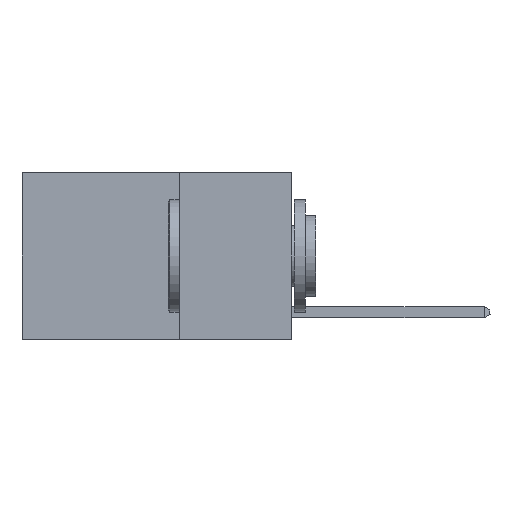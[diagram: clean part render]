
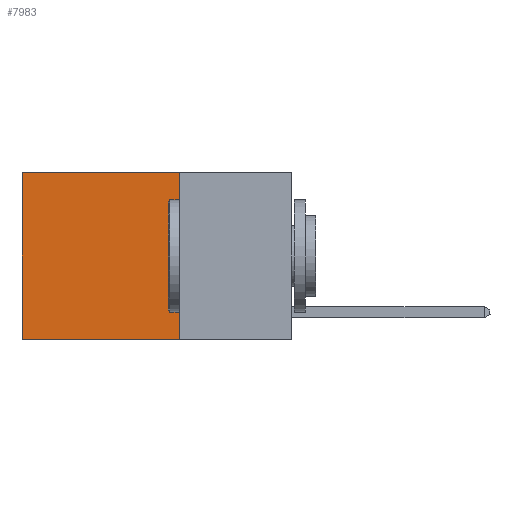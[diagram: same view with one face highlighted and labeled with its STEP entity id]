
A CAD part, left-side view. The second image highlights one B-rep face of the part: STEP entity #7983.
In plain terms, the highlighted planar face has unit normal (-1, 0, 0).
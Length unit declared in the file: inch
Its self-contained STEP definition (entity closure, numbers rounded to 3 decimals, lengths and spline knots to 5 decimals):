
#146 = VECTOR ( 'NONE', #8504, 39.37008 ) ;
#1455 = LINE ( 'NONE', #8732, #4046 ) ;
#1481 = DIRECTION ( 'NONE',  ( 0., 0., -1. ) ) ;
#2478 = CARTESIAN_POINT ( 'NONE',  ( 0.2625, 0.25, -0.37 ) ) ;
#3124 = ORIENTED_EDGE ( 'NONE', *, *, #3927, .T. ) ;
#3312 = DIRECTION ( 'NONE',  ( 0., 1., 0. ) ) ;
#3406 = VERTEX_POINT ( 'NONE', #4712 ) ;
#3596 = CARTESIAN_POINT ( 'NONE',  ( 0.2625, 0.25, 0. ) ) ;
#3927 = EDGE_CURVE ( 'NONE', #11149, #3406, #1455, .T. ) ;
#3940 = EDGE_CURVE ( 'NONE', #4665, #3406, #10703, .T. ) ;
#4046 = VECTOR ( 'NONE', #11753, 39.37008 ) ;
#4150 = CARTESIAN_POINT ( 'NONE',  ( 0.2625, 0.25, -0.37 ) ) ;
#4283 = EDGE_CURVE ( 'NONE', #8432, #4665, #7942, .T. ) ;
#4318 = CARTESIAN_POINT ( 'NONE',  ( 0.2625, 0.25, 0. ) ) ;
#4575 = DIRECTION ( 'NONE',  ( 1., 0., 0. ) ) ;
#4665 = VERTEX_POINT ( 'NONE', #4150 ) ;
#4712 = CARTESIAN_POINT ( 'NONE',  ( 0.2625, 0.6, -0.37 ) ) ;
#5341 = CARTESIAN_POINT ( 'NONE',  ( 0.2625, 0.6, 0. ) ) ;
#5641 = DIRECTION ( 'NONE',  ( 0., 1., 0. ) ) ;
#6466 = AXIS2_PLACEMENT_3D ( 'NONE', #10931, #4575, #1481 ) ;
#6627 = PLANE ( 'NONE',  #6466 ) ;
#6640 = ORIENTED_EDGE ( 'NONE', *, *, #3940, .F. ) ;
#6669 = VECTOR ( 'NONE', #5641, 39.37008 ) ;
#6754 = FACE_OUTER_BOUND ( 'NONE', #11500, .T. ) ;
#6976 = ORIENTED_EDGE ( 'NONE', *, *, #10155, .T. ) ;
#7942 = LINE ( 'NONE', #4318, #146 ) ;
#7983 = ADVANCED_FACE ( 'NONE', ( #6754 ), #6627, .F. ) ;
#8432 = VERTEX_POINT ( 'NONE', #3596 ) ;
#8504 = DIRECTION ( 'NONE',  ( 0., 0., -1. ) ) ;
#8730 = LINE ( 'NONE', #11819, #13344 ) ;
#8732 = CARTESIAN_POINT ( 'NONE',  ( 0.2625, 0.6, 0. ) ) ;
#10155 = EDGE_CURVE ( 'NONE', #8432, #11149, #8730, .T. ) ;
#10672 = ORIENTED_EDGE ( 'NONE', *, *, #4283, .F. ) ;
#10703 = LINE ( 'NONE', #2478, #6669 ) ;
#10931 = CARTESIAN_POINT ( 'NONE',  ( 0.2625, 0.25, 0. ) ) ;
#11149 = VERTEX_POINT ( 'NONE', #5341 ) ;
#11500 = EDGE_LOOP ( 'NONE', ( #3124, #6640, #10672, #6976 ) ) ;
#11753 = DIRECTION ( 'NONE',  ( 0., 0., -1. ) ) ;
#11819 = CARTESIAN_POINT ( 'NONE',  ( 0.2625, 0.25, 0. ) ) ;
#13344 = VECTOR ( 'NONE', #3312, 39.37008 ) ;
